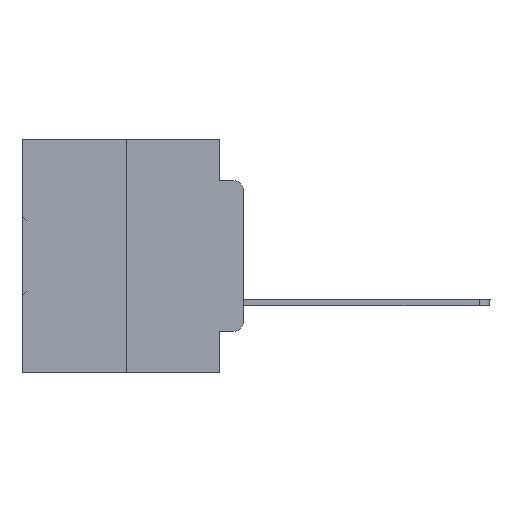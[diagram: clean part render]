
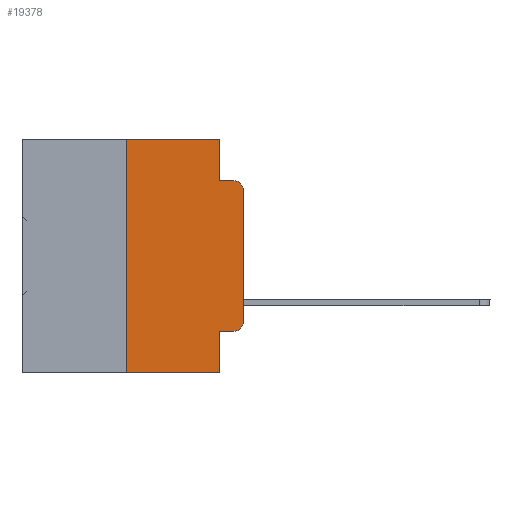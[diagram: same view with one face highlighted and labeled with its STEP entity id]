
A CAD part, left-side view. The second image highlights one B-rep face of the part: STEP entity #19378.
In plain terms, the highlighted planar face has unit normal (-1, 0, 0).
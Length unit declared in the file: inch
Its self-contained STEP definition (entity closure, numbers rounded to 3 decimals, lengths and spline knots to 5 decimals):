
#310 = ORIENTED_EDGE ( 'NONE', *, *, #18360, .T. ) ;
#1421 = VECTOR ( 'NONE', #4559, 39.37008 ) ;
#1714 = LINE ( 'NONE', #13383, #21336 ) ;
#2357 = CIRCLE ( 'NONE', #15161, 0.02 ) ;
#2643 = DIRECTION ( 'NONE',  ( 0., 0., -1. ) ) ;
#2832 = VERTEX_POINT ( 'NONE', #30587 ) ;
#2995 = VERTEX_POINT ( 'NONE', #25843 ) ;
#3363 = VERTEX_POINT ( 'NONE', #14512 ) ;
#3604 = LINE ( 'NONE', #25807, #4681 ) ;
#3974 = VERTEX_POINT ( 'NONE', #30245 ) ;
#4473 = LINE ( 'NONE', #31964, #23319 ) ;
#4559 = DIRECTION ( 'NONE',  ( 0., -1., 0. ) ) ;
#4665 = DIRECTION ( 'NONE',  ( 0., 0., -1. ) ) ;
#4681 = VECTOR ( 'NONE', #11984, 39.37008 ) ;
#5011 = ORIENTED_EDGE ( 'NONE', *, *, #5392, .F. ) ;
#5392 = EDGE_CURVE ( 'NONE', #15796, #2832, #33496, .T. ) ;
#5902 = ORIENTED_EDGE ( 'NONE', *, *, #34481, .F. ) ;
#6874 = DIRECTION ( 'NONE',  ( 0., 0., -1. ) ) ;
#7719 = DIRECTION ( 'NONE',  ( 0., -1., 0. ) ) ;
#7838 = CARTESIAN_POINT ( 'NONE',  ( 0., 0.473, -0.5 ) ) ;
#8633 = EDGE_CURVE ( 'NONE', #2995, #3974, #4473, .T. ) ;
#9076 = CARTESIAN_POINT ( 'NONE',  ( 0., 0.051, -0.5 ) ) ;
#9217 = DIRECTION ( 'NONE',  ( -1., 0., 0. ) ) ;
#10953 = VECTOR ( 'NONE', #6874, 39.37008 ) ;
#10963 = ORIENTED_EDGE ( 'NONE', *, *, #24654, .F. ) ;
#11194 = ORIENTED_EDGE ( 'NONE', *, *, #19246, .F. ) ;
#11198 = PLANE ( 'NONE',  #31709 ) ;
#11624 = AXIS2_PLACEMENT_3D ( 'NONE', #30875, #9217, #14692 ) ;
#11701 = CARTESIAN_POINT ( 'NONE',  ( 0., 0.02, -0.4115 ) ) ;
#11984 = DIRECTION ( 'NONE',  ( 0., -1., 0. ) ) ;
#12202 = CIRCLE ( 'NONE', #11624, 0.02 ) ;
#12889 = LINE ( 'NONE', #34322, #10953 ) ;
#13372 = VECTOR ( 'NONE', #30782, 39.37008 ) ;
#13383 = CARTESIAN_POINT ( 'NONE',  ( 0., 0.051, -0.4115 ) ) ;
#13590 = CARTESIAN_POINT ( 'NONE',  ( 0., 0.473, 0. ) ) ;
#13691 = ORIENTED_EDGE ( 'NONE', *, *, #24956, .T. ) ;
#13694 = CARTESIAN_POINT ( 'NONE',  ( 0., 0.051, -0.4115 ) ) ;
#14282 = VECTOR ( 'NONE', #4665, 39.37008 ) ;
#14512 = CARTESIAN_POINT ( 'NONE',  ( 0., 0.051, 0. ) ) ;
#14692 = DIRECTION ( 'NONE',  ( 0., 0., -1. ) ) ;
#14720 = VERTEX_POINT ( 'NONE', #13694 ) ;
#15120 = LINE ( 'NONE', #21105, #23006 ) ;
#15161 = AXIS2_PLACEMENT_3D ( 'NONE', #24212, #35111, #29473 ) ;
#15781 = DIRECTION ( 'NONE',  ( 0., 0., 1. ) ) ;
#15796 = VERTEX_POINT ( 'NONE', #34644 ) ;
#15868 = LINE ( 'NONE', #7838, #1421 ) ;
#15966 = LINE ( 'NONE', #32143, #14282 ) ;
#16504 = DIRECTION ( 'NONE',  ( 1., 0., 0. ) ) ;
#16537 = EDGE_LOOP ( 'NONE', ( #25552, #29395, #5011, #11194, #10963, #5902, #310, #16829, #30962, #13691 ) ) ;
#16829 = ORIENTED_EDGE ( 'NONE', *, *, #22191, .F. ) ;
#18360 = EDGE_CURVE ( 'NONE', #21278, #27625, #15868, .T. ) ;
#19246 = EDGE_CURVE ( 'NONE', #3363, #15796, #15966, .T. ) ;
#19378 = ADVANCED_FACE ( 'NONE', ( #33556 ), #11198, .F. ) ;
#20935 = EDGE_CURVE ( 'NONE', #14720, #21327, #1714, .T. ) ;
#21105 = CARTESIAN_POINT ( 'NONE',  ( 0., 0.25, 0. ) ) ;
#21278 = VERTEX_POINT ( 'NONE', #23156 ) ;
#21327 = VERTEX_POINT ( 'NONE', #11701 ) ;
#21336 = VECTOR ( 'NONE', #7719, 39.37008 ) ;
#22191 = EDGE_CURVE ( 'NONE', #14720, #27625, #12889, .T. ) ;
#23006 = VECTOR ( 'NONE', #31156, 39.37008 ) ;
#23156 = CARTESIAN_POINT ( 'NONE',  ( 0., 0.25, -0.5 ) ) ;
#23319 = VECTOR ( 'NONE', #15781, 39.37008 ) ;
#24212 = CARTESIAN_POINT ( 'NONE',  ( 0., 0.02, -0.1085 ) ) ;
#24654 = EDGE_CURVE ( 'NONE', #26986, #3363, #3604, .T. ) ;
#24956 = EDGE_CURVE ( 'NONE', #21327, #2995, #12202, .T. ) ;
#25552 = ORIENTED_EDGE ( 'NONE', *, *, #8633, .T. ) ;
#25807 = CARTESIAN_POINT ( 'NONE',  ( 0., 0.473, 0. ) ) ;
#25843 = CARTESIAN_POINT ( 'NONE',  ( 0., 0., -0.3915 ) ) ;
#26986 = VERTEX_POINT ( 'NONE', #29889 ) ;
#27332 = EDGE_CURVE ( 'NONE', #3974, #2832, #2357, .T. ) ;
#27625 = VERTEX_POINT ( 'NONE', #9076 ) ;
#28229 = CARTESIAN_POINT ( 'NONE',  ( 0., 0.051, -0.0885 ) ) ;
#29395 = ORIENTED_EDGE ( 'NONE', *, *, #27332, .T. ) ;
#29473 = DIRECTION ( 'NONE',  ( 0., 0., -1. ) ) ;
#29889 = CARTESIAN_POINT ( 'NONE',  ( 0., 0.25, 0. ) ) ;
#30245 = CARTESIAN_POINT ( 'NONE',  ( 0., 0., -0.1085 ) ) ;
#30587 = CARTESIAN_POINT ( 'NONE',  ( 0., 0.02, -0.0885 ) ) ;
#30782 = DIRECTION ( 'NONE',  ( 0., -1., 0. ) ) ;
#30875 = CARTESIAN_POINT ( 'NONE',  ( 0., 0.02, -0.3915 ) ) ;
#30962 = ORIENTED_EDGE ( 'NONE', *, *, #20935, .T. ) ;
#31156 = DIRECTION ( 'NONE',  ( 0., 0., 1. ) ) ;
#31709 = AXIS2_PLACEMENT_3D ( 'NONE', #13590, #16504, #2643 ) ;
#31964 = CARTESIAN_POINT ( 'NONE',  ( 0., 0., 0. ) ) ;
#32143 = CARTESIAN_POINT ( 'NONE',  ( 0., 0.051, 0. ) ) ;
#33496 = LINE ( 'NONE', #28229, #13372 ) ;
#33556 = FACE_OUTER_BOUND ( 'NONE', #16537, .T. ) ;
#34322 = CARTESIAN_POINT ( 'NONE',  ( 0., 0.051, 0. ) ) ;
#34481 = EDGE_CURVE ( 'NONE', #21278, #26986, #15120, .T. ) ;
#34644 = CARTESIAN_POINT ( 'NONE',  ( 0., 0.051, -0.0885 ) ) ;
#35111 = DIRECTION ( 'NONE',  ( -1., 0., 0. ) ) ;
